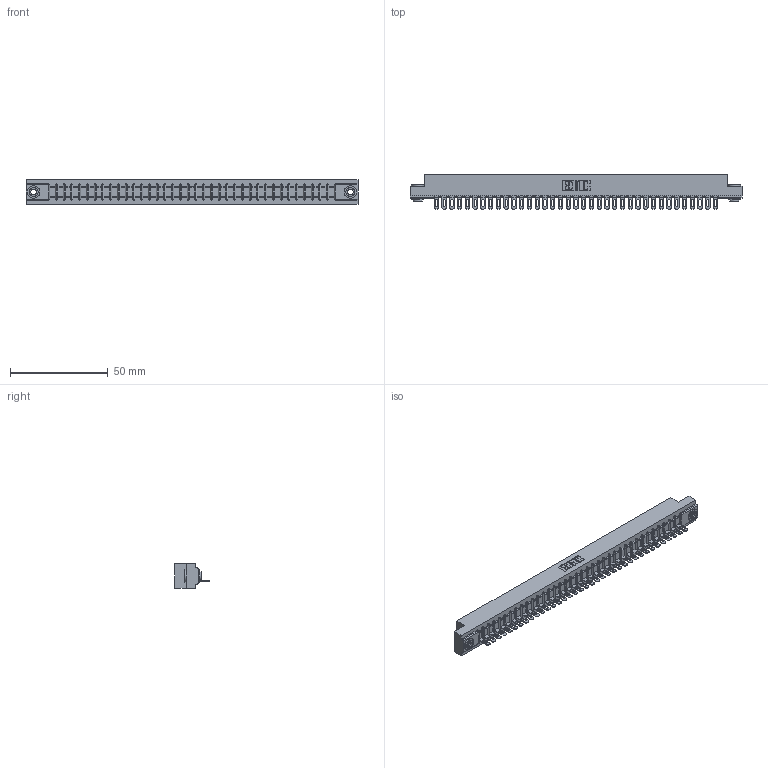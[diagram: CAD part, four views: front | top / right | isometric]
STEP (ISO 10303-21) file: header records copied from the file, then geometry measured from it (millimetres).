
FILE_DESCRIPTION (( 'STEP AP203' ), '1' );
FILE_NAME ('307-037-501-103.STEP', '2019-09-05T08:12:45', ( '' ), ( '' ), 'SwSTEP 2.0', 'SolidWorks 2016', '' );
FILE_SCHEMA (( 'CONFIG_CONTROL_DESIGN' ));
Length unit declared in the file: inch
Products named in the file (4): 345-250-002_345-250-002-102; 307-037-501-103; 307-290-002_501; 307 Part_.156 Dia Mounting Holes
Assembly tree (40 placements, depth 2):
  307-037-501-103
    307 Part_.156 Dia Mounting Holes
    307-290-002_501  x37
    345-250-002_345-250-002-102  x2
Bounding box: 169.62 x 17.42 x 12.7 mm (x, y, z)
Volume: 18147.9 mm3; surface area: 23208 mm2
Topology: 40 solids, 40 shells, 3020 faces, 9241 edges, 6054 vertices
Faces by surface type: plane 1722, cylinder 1214, sphere 76, cone 8
Entity records: 34195 total; most frequent: CARTESIAN_POINT 5745, ORIENTED_EDGE 5726, DIRECTION 5603, EDGE_CURVE 2863, VECTOR 2179, LINE 2179, VERTEX_POINT 1854, AXIS2_PLACEMENT_3D 1712
